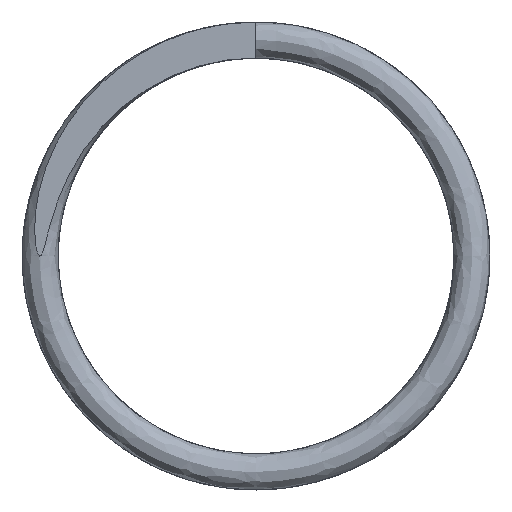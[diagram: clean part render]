
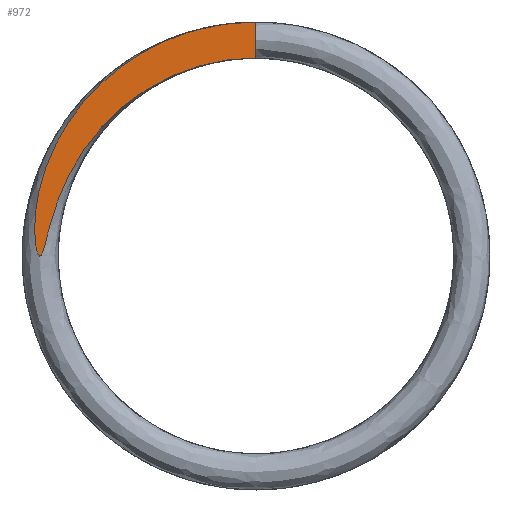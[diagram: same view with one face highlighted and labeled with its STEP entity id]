
A CAD part, front view. The second image highlights one B-rep face of the part: STEP entity #972.
In plain terms, the highlighted planar face has unit normal (0, -1, 0).
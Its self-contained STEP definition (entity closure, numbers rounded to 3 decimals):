
#6 = CARTESIAN_POINT ( 'NONE',  ( -5.618, 0., 1.222 ) ) ;
#20 = CARTESIAN_POINT ( 'NONE',  ( -6.046, 0., 0.033 ) ) ;
#34 = CARTESIAN_POINT ( 'NONE',  ( -5.467, 0., 3.29 ) ) ;
#45 = CARTESIAN_POINT ( 'NONE',  ( -0.787, 0., 6.463 ) ) ;
#164 = DIRECTION ( 'NONE',  ( 0., 0., 1. ) ) ;
#204 = VECTOR ( 'NONE', #1370, 1000. ) ;
#247 = LINE ( 'NONE', #2958, #204 ) ;
#267 = CARTESIAN_POINT ( 'NONE',  ( -1.583, 0., 5.291 ) ) ;
#281 = CARTESIAN_POINT ( 'NONE',  ( -5.779, 0., 0.644 ) ) ;
#294 = CARTESIAN_POINT ( 'NONE',  ( -6.083, 0., 0.126 ) ) ;
#309 = CARTESIAN_POINT ( 'NONE',  ( -5.16, 0., 3.793 ) ) ;
#321 = CARTESIAN_POINT ( 'NONE',  ( 0., 0., 6.5 ) ) ;
#547 = CARTESIAN_POINT ( 'NONE',  ( -2.684, 0., 4.847 ) ) ;
#562 = CARTESIAN_POINT ( 'NONE',  ( -5.875, 0., 0.254 ) ) ;
#576 = CARTESIAN_POINT ( 'NONE',  ( -6.114, 0., 0.272 ) ) ;
#589 = CARTESIAN_POINT ( 'NONE',  ( -4.556, 0., 4.559 ) ) ;
#651 = ORIENTED_EDGE ( 'NONE', *, *, #1539, .F. ) ;
#656 = ORIENTED_EDGE ( 'NONE', *, *, #1390, .F. ) ;
#796 = AXIS2_PLACEMENT_3D ( 'NONE', #3378, #1808, #164 ) ;
#826 = CARTESIAN_POINT ( 'NONE',  ( -3.678, 0., 4.181 ) ) ;
#839 = CARTESIAN_POINT ( 'NONE',  ( -5.921, 0., 0.112 ) ) ;
#853 = CARTESIAN_POINT ( 'NONE',  ( -6.139, 0., 0.467 ) ) ;
#865 = CARTESIAN_POINT ( 'NONE',  ( -3.67, 0., 5.333 ) ) ;
#906 = VERTEX_POINT ( 'NONE', #1275 ) ;
#972 = ADVANCED_FACE ( 'NONE', ( #1075 ), #1616, .F. ) ;
#1075 = FACE_OUTER_BOUND ( 'NONE', #1125, .T. ) ;
#1095 = CARTESIAN_POINT ( 'NONE',  ( 0., 0., 5.5 ) ) ;
#1107 = CARTESIAN_POINT ( 'NONE',  ( -4.517, 0., 3.33 ) ) ;
#1121 = CARTESIAN_POINT ( 'NONE',  ( -5.95, 0., 0.042 ) ) ;
#1125 = EDGE_LOOP ( 'NONE', ( #651, #656 ) ) ;
#1138 = CARTESIAN_POINT ( 'NONE',  ( -6.157, 0., 1.059 ) ) ;
#1151 = CARTESIAN_POINT ( 'NONE',  ( -2.663, 0., 5.923 ) ) ;
#1275 = CARTESIAN_POINT ( 'NONE',  ( 0., 0., 6.5 ) ) ;
#1370 = DIRECTION ( 'NONE',  ( 0., 0., -1. ) ) ;
#1383 = CARTESIAN_POINT ( 'NONE',  ( -5.169, 0., 2.335 ) ) ;
#1390 = EDGE_CURVE ( 'NONE', #906, #2323, #247, .T. ) ;
#1397 = CARTESIAN_POINT ( 'NONE',  ( -5.983, 0., 0.003 ) ) ;
#1411 = CARTESIAN_POINT ( 'NONE',  ( -5.933, 0., 2.209 ) ) ;
#1424 = CARTESIAN_POINT ( 'NONE',  ( -1.929, 0., 6.201 ) ) ;
#1539 = EDGE_CURVE ( 'NONE', #2323, #906, #3165, .T. ) ;
#1616 = PLANE ( 'NONE',  #796 ) ;
#1646 = CARTESIAN_POINT ( 'NONE',  ( -5.555, 0., 1.412 ) ) ;
#1660 = CARTESIAN_POINT ( 'NONE',  ( -6.02, 0., 0.006 ) ) ;
#1675 = CARTESIAN_POINT ( 'NONE',  ( -5.558, 0., 3.117 ) ) ;
#1686 = CARTESIAN_POINT ( 'NONE',  ( -1.362, 0., 6.354 ) ) ;
#1808 = DIRECTION ( 'NONE',  ( 0., 1., 0. ) ) ;
#1912 = CARTESIAN_POINT ( 'NONE',  ( -0.802, 0., 5.457 ) ) ;
#1926 = CARTESIAN_POINT ( 'NONE',  ( -5.73, 0., 0.838 ) ) ;
#1940 = CARTESIAN_POINT ( 'NONE',  ( -6.056, 0., 0.057 ) ) ;
#1954 = CARTESIAN_POINT ( 'NONE',  ( -5.269, 0., 3.628 ) ) ;
#1966 = CARTESIAN_POINT ( 'NONE',  ( -0.394, 0., 6.5 ) ) ;
#2183 = CARTESIAN_POINT ( 'NONE',  ( -1.959, 0., 5.168 ) ) ;
#2197 = CARTESIAN_POINT ( 'NONE',  ( -5.851, 0., 0.352 ) ) ;
#2211 = CARTESIAN_POINT ( 'NONE',  ( -6.094, 0., 0.175 ) ) ;
#2225 = CARTESIAN_POINT ( 'NONE',  ( -4.815, 0., 4.268 ) ) ;
#2238 = CARTESIAN_POINT ( 'NONE',  ( 0., 0., 5.5 ) ) ;
#2323 = VERTEX_POINT ( 'NONE', #2238 ) ;
#2454 = CARTESIAN_POINT ( 'NONE',  ( -3.035, 0., 4.645 ) ) ;
#2465 = CARTESIAN_POINT ( 'NONE',  ( -5.913, 0., 0.135 ) ) ;
#2480 = CARTESIAN_POINT ( 'NONE',  ( -6.121, 0., 0.32 ) ) ;
#2494 = CARTESIAN_POINT ( 'NONE',  ( -3.986, 0., 5.091 ) ) ;
#2718 = CARTESIAN_POINT ( 'NONE',  ( -3.974, 0., 3.919 ) ) ;
#2730 = CARTESIAN_POINT ( 'NONE',  ( -5.94, 0., 0.065 ) ) ;
#2742 = CARTESIAN_POINT ( 'NONE',  ( -6.145, 0., 0.565 ) ) ;
#2754 = CARTESIAN_POINT ( 'NONE',  ( -3.01, 0., 5.747 ) ) ;
#2958 = CARTESIAN_POINT ( 'NONE',  ( 0., 0., 6.5 ) ) ;
#2970 = CARTESIAN_POINT ( 'NONE',  ( -4.756, 0., 3.011 ) ) ;
#2983 = CARTESIAN_POINT ( 'NONE',  ( -5.973, 0., 0.012 ) ) ;
#2995 = CARTESIAN_POINT ( 'NONE',  ( -6.108, 0., 1.447 ) ) ;
#3008 = CARTESIAN_POINT ( 'NONE',  ( -2.116, 0., 6.137 ) ) ;
#3165 = B_SPLINE_CURVE_WITH_KNOTS ( 'NONE', 3,
 ( #1095, #3475, #1912, #267, #2183, #547, #2454, #826, #2718, #1107, #2970, #1383, #3223, #1646, #6, #1926, #281, #2197, #562, #2465, #839, #2730, #1121, #2983, #1397, #3238, #1660, #20, #1940, #294, #2211, #576, #2480, #853, #2742, #1138, #2995, #1411, #3252, #1675, #34, #1954, #309, #2225, #589, #2494, #865, #2754, #1151, #3008, #1424, #3265, #1686, #45, #1966, #321 ),
 .UNSPECIFIED., .F., .F.,
 ( 4, 2, 2, 2, 2, 2, 2, 2, 2, 2, 2, 2, 2, 2, 2, 2, 2, 2, 2, 2, 2, 2, 2, 2, 2, 2, 2, 4 ),
 ( 0., 0.001, 0.002, 0.004, 0.005, 0.006, 0.007, 0.008, 0.008, 0.009, 0.009, 0.009, 0.009, 0.009, 0.009, 0.009, 0.009, 0.01, 0.011, 0.012, 0.013, 0.013, 0.014, 0.016, 0.017, 0.017, 0.018, 0.019 ),
 .UNSPECIFIED. ) ;
#3223 = CARTESIAN_POINT ( 'NONE',  ( -5.343, 0., 1.974 ) ) ;
#3238 = CARTESIAN_POINT ( 'NONE',  ( -6.008, 0., -0.002 ) ) ;
#3252 = CARTESIAN_POINT ( 'NONE',  ( -5.803, 0., 2.585 ) ) ;
#3265 = CARTESIAN_POINT ( 'NONE',  ( -1.552, 0., 6.309 ) ) ;
#3378 = CARTESIAN_POINT ( 'NONE',  ( 0., 0., 0. ) ) ;
#3475 = CARTESIAN_POINT ( 'NONE',  ( -0.401, 0., 5.5 ) ) ;
